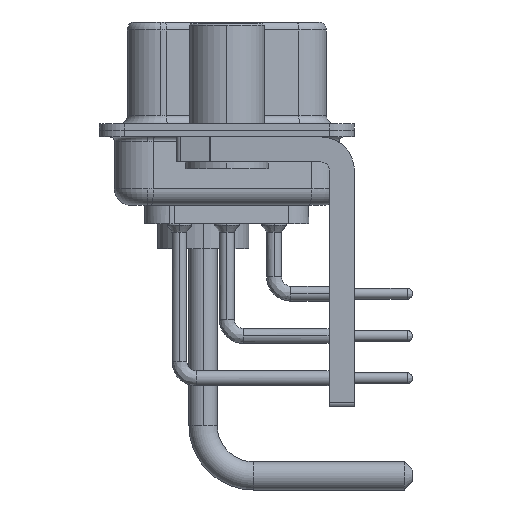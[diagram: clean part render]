
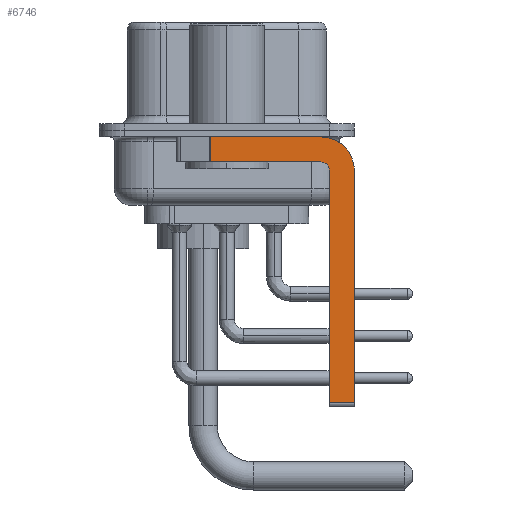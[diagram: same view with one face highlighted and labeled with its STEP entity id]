
A CAD part, left-side view. The second image highlights one B-rep face of the part: STEP entity #6746.
In plain terms, the highlighted planar face has unit normal (-1, 0, 0).
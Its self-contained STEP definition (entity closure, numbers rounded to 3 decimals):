
#21 = EDGE_CURVE ( 'NONE', #18985, #34060, #35980, .T. ) ;
#60 = CARTESIAN_POINT ( 'NONE',  ( -2.9, -6.15, -16.35 ) ) ;
#209 = VERTEX_POINT ( 'NONE', #36953 ) ;
#1158 = CARTESIAN_POINT ( 'NONE',  ( -2.9, -5.65, -2.4 ) ) ;
#1489 = EDGE_CURVE ( 'NONE', #209, #4832, #37537, .T. ) ;
#1721 = VERTEX_POINT ( 'NONE', #60 ) ;
#2897 = CARTESIAN_POINT ( 'NONE',  ( -2.9, -5.65, -2.4 ) ) ;
#3086 = DIRECTION ( 'NONE',  ( -1., 0., 0. ) ) ;
#3192 = CIRCLE ( 'NONE', #28246, 0.5 ) ;
#3609 = PLANE ( 'NONE',  #17644 ) ;
#3798 = FACE_OUTER_BOUND ( 'NONE', #22325, .T. ) ;
#3947 = DIRECTION ( 'NONE',  ( 0., 1., 0. ) ) ;
#4222 = CARTESIAN_POINT ( 'NONE',  ( -2.9, -7.65, -16.35 ) ) ;
#4832 = VERTEX_POINT ( 'NONE', #4222 ) ;
#5239 = CARTESIAN_POINT ( 'NONE',  ( -2.9, 0.978, -1.9 ) ) ;
#6148 = EDGE_CURVE ( 'NONE', #21812, #28155, #3192, .T. ) ;
#6746 = ADVANCED_FACE ( 'NONE', ( #3798 ), #3609, .F. ) ;
#7745 = CARTESIAN_POINT ( 'NONE',  ( -2.9, -6.15, -16.6 ) ) ;
#10022 = CARTESIAN_POINT ( 'NONE',  ( -2.9, -5.65, -1.9 ) ) ;
#10067 = DIRECTION ( 'NONE',  ( 1., 0., 0. ) ) ;
#12029 = VECTOR ( 'NONE', #30519, 1000. ) ;
#12493 = DIRECTION ( 'NONE',  ( 0., 0., 1. ) ) ;
#12685 = ORIENTED_EDGE ( 'NONE', *, *, #13874, .F. ) ;
#12899 = DIRECTION ( 'NONE',  ( 0., 0., 1. ) ) ;
#12968 = CIRCLE ( 'NONE', #34839, 2. ) ;
#13095 = LINE ( 'NONE', #7745, #38598 ) ;
#13228 = CARTESIAN_POINT ( 'NONE',  ( -2.9, -5.65, -2.4 ) ) ;
#13705 = DIRECTION ( 'NONE',  ( 0., 0., -1. ) ) ;
#13874 = EDGE_CURVE ( 'NONE', #28155, #35489, #30846, .T. ) ;
#14820 = CARTESIAN_POINT ( 'NONE',  ( -2.9, -5.65, -0.4 ) ) ;
#15336 = VECTOR ( 'NONE', #16765, 1000. ) ;
#15415 = CARTESIAN_POINT ( 'NONE',  ( -2.9, 3., -0.4 ) ) ;
#15578 = EDGE_CURVE ( 'NONE', #1721, #21812, #13095, .T. ) ;
#16765 = DIRECTION ( 'NONE',  ( 0., 0., -1. ) ) ;
#17131 = ORIENTED_EDGE ( 'NONE', *, *, #6148, .F. ) ;
#17644 = AXIS2_PLACEMENT_3D ( 'NONE', #13228, #10067, #22430 ) ;
#18269 = ORIENTED_EDGE ( 'NONE', *, *, #1489, .F. ) ;
#18985 = VERTEX_POINT ( 'NONE', #26137 ) ;
#19750 = CARTESIAN_POINT ( 'NONE',  ( -2.9, -5.65, -16.35 ) ) ;
#21812 = VERTEX_POINT ( 'NONE', #29059 ) ;
#22111 = LINE ( 'NONE', #19750, #28818 ) ;
#22325 = EDGE_LOOP ( 'NONE', ( #35496, #29984, #12685, #17131, #37329, #28559, #18269, #32102 ) ) ;
#22430 = DIRECTION ( 'NONE',  ( 0., 0., -1. ) ) ;
#23309 = LINE ( 'NONE', #5239, #30443 ) ;
#23593 = VECTOR ( 'NONE', #3947, 1000. ) ;
#25827 = CARTESIAN_POINT ( 'NONE',  ( -2.9, -5.65, -1.9 ) ) ;
#25836 = DIRECTION ( 'NONE',  ( 0., -1., 0. ) ) ;
#26137 = CARTESIAN_POINT ( 'NONE',  ( -2.9, 0.978, -0.4 ) ) ;
#26260 = EDGE_CURVE ( 'NONE', #18985, #35489, #23309, .T. ) ;
#28155 = VERTEX_POINT ( 'NONE', #25827 ) ;
#28246 = AXIS2_PLACEMENT_3D ( 'NONE', #2897, #3086, #12493 ) ;
#28559 = ORIENTED_EDGE ( 'NONE', *, *, #32250, .T. ) ;
#28818 = VECTOR ( 'NONE', #25836, 1000. ) ;
#28953 = EDGE_CURVE ( 'NONE', #34060, #209, #12968, .T. ) ;
#29059 = CARTESIAN_POINT ( 'NONE',  ( -2.9, -6.15, -2.4 ) ) ;
#29984 = ORIENTED_EDGE ( 'NONE', *, *, #26260, .T. ) ;
#30443 = VECTOR ( 'NONE', #13705, 1000. ) ;
#30519 = DIRECTION ( 'NONE',  ( 0., -1., 0. ) ) ;
#30846 = LINE ( 'NONE', #10022, #23593 ) ;
#32102 = ORIENTED_EDGE ( 'NONE', *, *, #28953, .F. ) ;
#32250 = EDGE_CURVE ( 'NONE', #1721, #4832, #22111, .T. ) ;
#34060 = VERTEX_POINT ( 'NONE', #14820 ) ;
#34569 = CARTESIAN_POINT ( 'NONE',  ( -2.9, -7.65, -2.4 ) ) ;
#34839 = AXIS2_PLACEMENT_3D ( 'NONE', #1158, #36847, #37613 ) ;
#35489 = VERTEX_POINT ( 'NONE', #37325 ) ;
#35496 = ORIENTED_EDGE ( 'NONE', *, *, #21, .F. ) ;
#35980 = LINE ( 'NONE', #15415, #12029 ) ;
#36847 = DIRECTION ( 'NONE',  ( 1., 0., 0. ) ) ;
#36953 = CARTESIAN_POINT ( 'NONE',  ( -2.9, -7.65, -2.4 ) ) ;
#37325 = CARTESIAN_POINT ( 'NONE',  ( -2.9, 0.978, -1.9 ) ) ;
#37329 = ORIENTED_EDGE ( 'NONE', *, *, #15578, .F. ) ;
#37537 = LINE ( 'NONE', #34569, #15336 ) ;
#37613 = DIRECTION ( 'NONE',  ( 0., 0., -1. ) ) ;
#38598 = VECTOR ( 'NONE', #12899, 1000. ) ;
